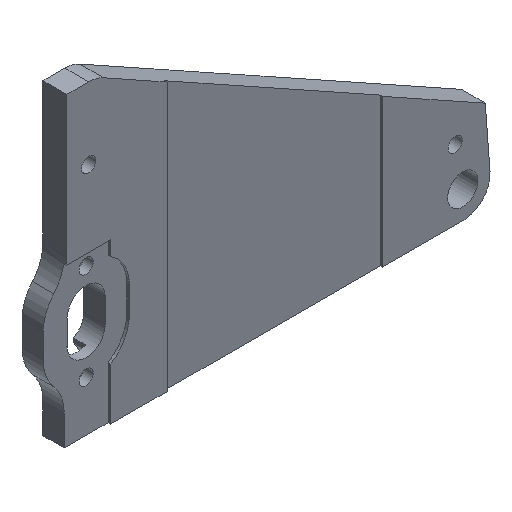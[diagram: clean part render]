
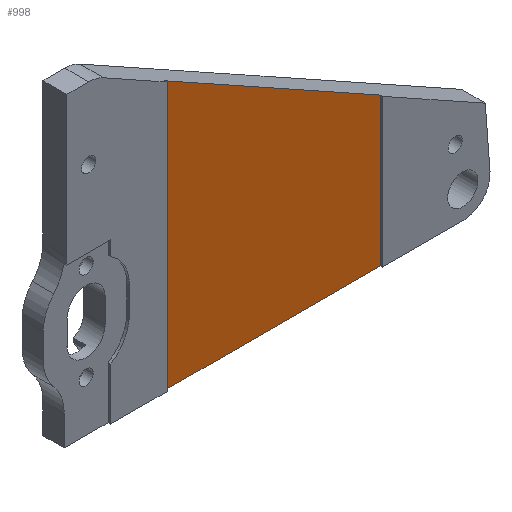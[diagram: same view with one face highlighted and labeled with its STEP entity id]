
A CAD part, isometric view. The second image highlights one B-rep face of the part: STEP entity #998.
In plain terms, the highlighted planar face has unit normal (0, -1, 0).
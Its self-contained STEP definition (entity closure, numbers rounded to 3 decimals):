
#21 = ORIENTED_EDGE ( 'NONE', *, *, #274, .F. ) ;
#57 = LINE ( 'NONE', #1517, #1752 ) ;
#254 = PLANE ( 'NONE',  #2091 ) ;
#274 = EDGE_CURVE ( 'NONE', #1466, #883, #346, .T. ) ;
#303 = DIRECTION ( 'NONE',  ( 1., 0., 0. ) ) ;
#326 = CARTESIAN_POINT ( 'NONE',  ( 66.167, 0.457, 0. ) ) ;
#346 = LINE ( 'NONE', #797, #2042 ) ;
#427 = CARTESIAN_POINT ( 'NONE',  ( 0., 0.457, 0. ) ) ;
#479 = CARTESIAN_POINT ( 'NONE',  ( 66.167, 0.457, -33.41 ) ) ;
#552 = CARTESIAN_POINT ( 'NONE',  ( 21.006, 0.457, -8.229 ) ) ;
#584 = DIRECTION ( 'NONE',  ( 0., 1., 0. ) ) ;
#629 = VERTEX_POINT ( 'NONE', #479 ) ;
#652 = ORIENTED_EDGE ( 'NONE', *, *, #1142, .T. ) ;
#704 = VERTEX_POINT ( 'NONE', #1997 ) ;
#797 = CARTESIAN_POINT ( 'NONE',  ( 21.006, 0.457, 0. ) ) ;
#883 = VERTEX_POINT ( 'NONE', #552 ) ;
#998 = ADVANCED_FACE ( 'NONE', ( #1320 ), #254, .F. ) ;
#1052 = VECTOR ( 'NONE', #303, 1000. ) ;
#1137 = DIRECTION ( 'NONE',  ( 0., 0., 1. ) ) ;
#1142 = EDGE_CURVE ( 'NONE', #1466, #704, #1453, .T. ) ;
#1230 = EDGE_CURVE ( 'NONE', #704, #629, #1342, .T. ) ;
#1291 = CARTESIAN_POINT ( 'NONE',  ( 0., 0.457, -64.364 ) ) ;
#1320 = FACE_OUTER_BOUND ( 'NONE', #1732, .T. ) ;
#1338 = ORIENTED_EDGE ( 'NONE', *, *, #1379, .T. ) ;
#1342 = LINE ( 'NONE', #326, #1681 ) ;
#1360 = CARTESIAN_POINT ( 'NONE',  ( 21.006, 0.457, -64.364 ) ) ;
#1379 = EDGE_CURVE ( 'NONE', #629, #883, #57, .T. ) ;
#1453 = LINE ( 'NONE', #1291, #1052 ) ;
#1466 = VERTEX_POINT ( 'NONE', #1360 ) ;
#1517 = CARTESIAN_POINT ( 'NONE',  ( 1.482, 0.457, 2.657 ) ) ;
#1681 = VECTOR ( 'NONE', #1137, 1000. ) ;
#1683 = DIRECTION ( 'NONE',  ( -0.873, 0., 0.487 ) ) ;
#1732 = EDGE_LOOP ( 'NONE', ( #1942, #1338, #21, #652 ) ) ;
#1742 = DIRECTION ( 'NONE',  ( 0., 0., 1. ) ) ;
#1752 = VECTOR ( 'NONE', #1683, 1000. ) ;
#1942 = ORIENTED_EDGE ( 'NONE', *, *, #1230, .T. ) ;
#1997 = CARTESIAN_POINT ( 'NONE',  ( 66.167, 0.457, -64.364 ) ) ;
#2042 = VECTOR ( 'NONE', #2087, 1000. ) ;
#2087 = DIRECTION ( 'NONE',  ( 0., 0., 1. ) ) ;
#2091 = AXIS2_PLACEMENT_3D ( 'NONE', #427, #584, #1742 ) ;
